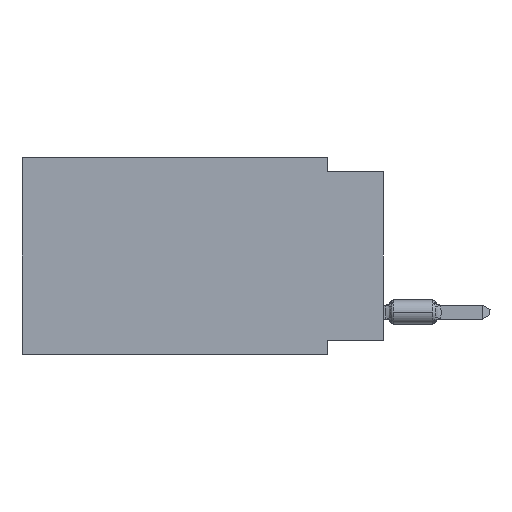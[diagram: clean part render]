
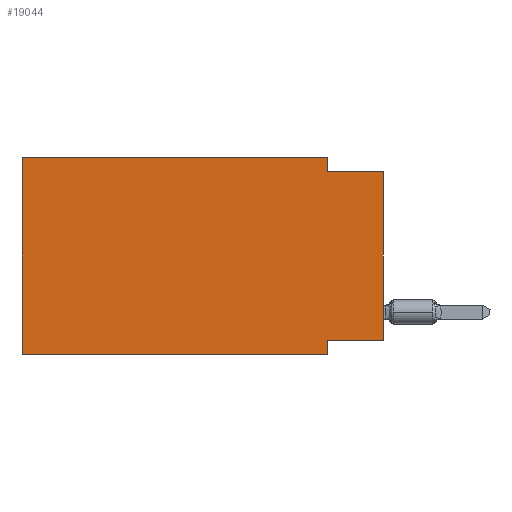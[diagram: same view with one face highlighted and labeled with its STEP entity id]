
A CAD part, left-side view. The second image highlights one B-rep face of the part: STEP entity #19044.
In plain terms, the highlighted planar face has unit normal (-1, 0, 0).
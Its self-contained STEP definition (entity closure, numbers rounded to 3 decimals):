
#121 = VERTEX_POINT ( 'NONE', #17081 ) ;
#178 = EDGE_CURVE ( 'NONE', #12832, #3881, #29310, .T. ) ;
#864 = ORIENTED_EDGE ( 'NONE', *, *, #32229, .F. ) ;
#1499 = CARTESIAN_POINT ( 'NONE',  ( 0., 2.54, -8.255 ) ) ;
#3022 = DIRECTION ( 'NONE',  ( 0., 0., 1. ) ) ;
#3881 = VERTEX_POINT ( 'NONE', #25842 ) ;
#4081 = VECTOR ( 'NONE', #43337, 1000. ) ;
#4531 = EDGE_CURVE ( 'NONE', #47677, #3881, #34910, .T. ) ;
#6633 = ORIENTED_EDGE ( 'NONE', *, *, #28472, .F. ) ;
#6766 = DIRECTION ( 'NONE',  ( 0., -1., 0. ) ) ;
#6773 = DIRECTION ( 'NONE',  ( 1., 0., 0. ) ) ;
#8881 = DIRECTION ( 'NONE',  ( 0., 1., 0. ) ) ;
#9540 = CARTESIAN_POINT ( 'NONE',  ( 0., 0., -8.255 ) ) ;
#10499 = VECTOR ( 'NONE', #17345, 1000. ) ;
#11507 = VECTOR ( 'NONE', #3022, 1000. ) ;
#12113 = DIRECTION ( 'NONE',  ( 0., 0., -1. ) ) ;
#12153 = ORIENTED_EDGE ( 'NONE', *, *, #16165, .F. ) ;
#12481 = VECTOR ( 'NONE', #6766, 1000. ) ;
#12832 = VERTEX_POINT ( 'NONE', #1499 ) ;
#15559 = EDGE_CURVE ( 'NONE', #51184, #12832, #32543, .T. ) ;
#16138 = DIRECTION ( 'NONE',  ( 0., -1., 0. ) ) ;
#16165 = EDGE_CURVE ( 'NONE', #51021, #22439, #31119, .T. ) ;
#16462 = PLANE ( 'NONE',  #37937 ) ;
#17081 = CARTESIAN_POINT ( 'NONE',  ( 0., 2.54, 0. ) ) ;
#17345 = DIRECTION ( 'NONE',  ( 0., 0., -1. ) ) ;
#17476 = DIRECTION ( 'NONE',  ( 0., 0., 1. ) ) ;
#18393 = CARTESIAN_POINT ( 'NONE',  ( 0., 2.54, 0. ) ) ;
#18465 = LINE ( 'NONE', #43972, #12481 ) ;
#19044 = ADVANCED_FACE ( 'NONE', ( #49309 ), #16462, .F. ) ;
#19232 = ORIENTED_EDGE ( 'NONE', *, *, #4531, .T. ) ;
#19583 = LINE ( 'NONE', #35352, #11507 ) ;
#21090 = VECTOR ( 'NONE', #17476, 1000. ) ;
#21158 = CARTESIAN_POINT ( 'NONE',  ( 0., 2.54, -8.89 ) ) ;
#21296 = CARTESIAN_POINT ( 'NONE',  ( 0., 0., 0. ) ) ;
#21552 = VECTOR ( 'NONE', #16138, 1000. ) ;
#22439 = VERTEX_POINT ( 'NONE', #38765 ) ;
#24768 = CARTESIAN_POINT ( 'NONE',  ( 0., 16.383, 0. ) ) ;
#25656 = ORIENTED_EDGE ( 'NONE', *, *, #34981, .T. ) ;
#25842 = CARTESIAN_POINT ( 'NONE',  ( 0., 2.54, -8.89 ) ) ;
#26843 = EDGE_CURVE ( 'NONE', #47677, #39402, #19583, .T. ) ;
#28472 = EDGE_CURVE ( 'NONE', #39402, #121, #18465, .T. ) ;
#29206 = VECTOR ( 'NONE', #8881, 1000. ) ;
#29310 = LINE ( 'NONE', #21158, #10499 ) ;
#30863 = CARTESIAN_POINT ( 'NONE',  ( 0., 0., -0.635 ) ) ;
#31119 = LINE ( 'NONE', #30863, #4081 ) ;
#32229 = EDGE_CURVE ( 'NONE', #121, #51021, #36484, .T. ) ;
#32543 = LINE ( 'NONE', #46077, #29206 ) ;
#34533 = ORIENTED_EDGE ( 'NONE', *, *, #178, .F. ) ;
#34910 = LINE ( 'NONE', #51473, #21552 ) ;
#34963 = DIRECTION ( 'NONE',  ( 0., 0., -1. ) ) ;
#34981 = EDGE_CURVE ( 'NONE', #51184, #22439, #53417, .T. ) ;
#35352 = CARTESIAN_POINT ( 'NONE',  ( 0., 16.383, 0. ) ) ;
#36484 = LINE ( 'NONE', #18393, #52129 ) ;
#37937 = AXIS2_PLACEMENT_3D ( 'NONE', #39899, #6773, #12113 ) ;
#38765 = CARTESIAN_POINT ( 'NONE',  ( 0., 0., -0.635 ) ) ;
#39402 = VERTEX_POINT ( 'NONE', #24768 ) ;
#39899 = CARTESIAN_POINT ( 'NONE',  ( 0., 16.383, 0. ) ) ;
#41102 = ORIENTED_EDGE ( 'NONE', *, *, #26843, .F. ) ;
#41339 = CARTESIAN_POINT ( 'NONE',  ( 0., 2.54, -0.635 ) ) ;
#42426 = CARTESIAN_POINT ( 'NONE',  ( 0., 16.383, -8.89 ) ) ;
#43337 = DIRECTION ( 'NONE',  ( 0., -1., 0. ) ) ;
#43374 = EDGE_LOOP ( 'NONE', ( #25656, #12153, #864, #6633, #41102, #19232, #34533, #51687 ) ) ;
#43972 = CARTESIAN_POINT ( 'NONE',  ( 0., 16.383, 0. ) ) ;
#46077 = CARTESIAN_POINT ( 'NONE',  ( 0., 0., -8.255 ) ) ;
#47677 = VERTEX_POINT ( 'NONE', #42426 ) ;
#49309 = FACE_OUTER_BOUND ( 'NONE', #43374, .T. ) ;
#51021 = VERTEX_POINT ( 'NONE', #41339 ) ;
#51184 = VERTEX_POINT ( 'NONE', #9540 ) ;
#51473 = CARTESIAN_POINT ( 'NONE',  ( 0., 16.383, -8.89 ) ) ;
#51687 = ORIENTED_EDGE ( 'NONE', *, *, #15559, .F. ) ;
#52129 = VECTOR ( 'NONE', #34963, 1000. ) ;
#53417 = LINE ( 'NONE', #21296, #21090 ) ;
